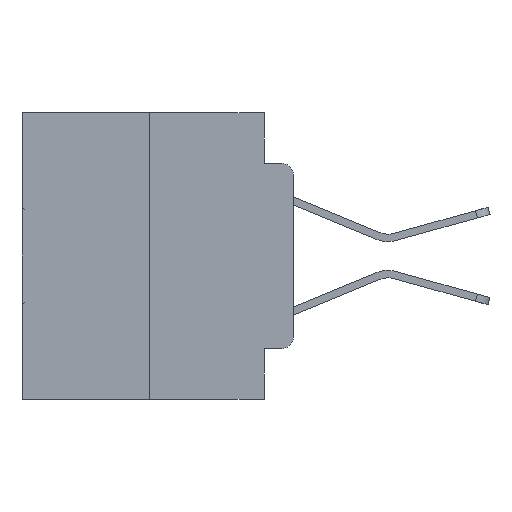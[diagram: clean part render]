
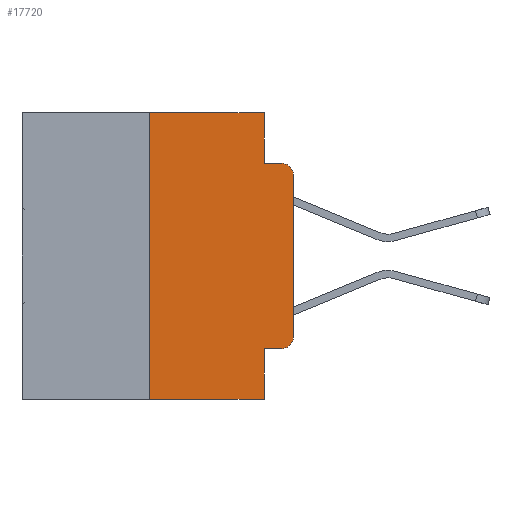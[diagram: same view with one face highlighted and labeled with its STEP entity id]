
A CAD part, left-side view. The second image highlights one B-rep face of the part: STEP entity #17720.
In plain terms, the highlighted planar face has unit normal (-1, 0, 0).
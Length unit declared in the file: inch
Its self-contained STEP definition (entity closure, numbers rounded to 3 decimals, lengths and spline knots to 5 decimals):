
#179 = EDGE_CURVE ( 'NONE', #6998, #27669, #27585, .T. ) ;
#765 = CARTESIAN_POINT ( 'NONE',  ( 0., 0.473, 0. ) ) ;
#1278 = DIRECTION ( 'NONE',  ( 0., -1., 0. ) ) ;
#1785 = CARTESIAN_POINT ( 'NONE',  ( 0., 0.051, -0.0885 ) ) ;
#2516 = VECTOR ( 'NONE', #15667, 39.37008 ) ;
#3267 = DIRECTION ( 'NONE',  ( 1., 0., 0. ) ) ;
#3466 = CARTESIAN_POINT ( 'NONE',  ( 0., 0.051, 0. ) ) ;
#3593 = FACE_OUTER_BOUND ( 'NONE', #20076, .T. ) ;
#4179 = CARTESIAN_POINT ( 'NONE',  ( 0., 0.051, 0. ) ) ;
#4192 = CARTESIAN_POINT ( 'NONE',  ( 0., 0.02, -0.0885 ) ) ;
#4273 = CARTESIAN_POINT ( 'NONE',  ( 0., 0.051, -0.4115 ) ) ;
#4845 = VERTEX_POINT ( 'NONE', #1785 ) ;
#4847 = VECTOR ( 'NONE', #18479, 39.37008 ) ;
#4852 = VERTEX_POINT ( 'NONE', #4273 ) ;
#5198 = ORIENTED_EDGE ( 'NONE', *, *, #9910, .T. ) ;
#5583 = VERTEX_POINT ( 'NONE', #18699 ) ;
#5789 = DIRECTION ( 'NONE',  ( -1., 0., 0. ) ) ;
#6091 = VERTEX_POINT ( 'NONE', #9246 ) ;
#6861 = VERTEX_POINT ( 'NONE', #4192 ) ;
#6998 = VERTEX_POINT ( 'NONE', #18765 ) ;
#7074 = VECTOR ( 'NONE', #29025, 39.37008 ) ;
#7220 = VERTEX_POINT ( 'NONE', #7951 ) ;
#7822 = ORIENTED_EDGE ( 'NONE', *, *, #179, .F. ) ;
#7951 = CARTESIAN_POINT ( 'NONE',  ( 0., 0., -0.3915 ) ) ;
#8272 = LINE ( 'NONE', #4179, #13891 ) ;
#8754 = LINE ( 'NONE', #10656, #20482 ) ;
#9017 = DIRECTION ( 'NONE',  ( 0., 0., -1. ) ) ;
#9246 = CARTESIAN_POINT ( 'NONE',  ( 0., 0., -0.1085 ) ) ;
#9327 = ORIENTED_EDGE ( 'NONE', *, *, #19332, .F. ) ;
#9339 = AXIS2_PLACEMENT_3D ( 'NONE', #765, #3267, #19824 ) ;
#9910 = EDGE_CURVE ( 'NONE', #12800, #7220, #11887, .T. ) ;
#10075 = ORIENTED_EDGE ( 'NONE', *, *, #17796, .F. ) ;
#10470 = VERTEX_POINT ( 'NONE', #27005 ) ;
#10656 = CARTESIAN_POINT ( 'NONE',  ( 0., 0.25, 0. ) ) ;
#11222 = AXIS2_PLACEMENT_3D ( 'NONE', #11922, #28230, #14347 ) ;
#11785 = VECTOR ( 'NONE', #22159, 39.37008 ) ;
#11887 = CIRCLE ( 'NONE', #29180, 0.02 ) ;
#11922 = CARTESIAN_POINT ( 'NONE',  ( 0., 0.02, -0.1085 ) ) ;
#12688 = ORIENTED_EDGE ( 'NONE', *, *, #22464, .F. ) ;
#12800 = VERTEX_POINT ( 'NONE', #26592 ) ;
#13409 = LINE ( 'NONE', #17479, #7074 ) ;
#13891 = VECTOR ( 'NONE', #9017, 39.37008 ) ;
#14347 = DIRECTION ( 'NONE',  ( 0., 0., -1. ) ) ;
#14672 = CARTESIAN_POINT ( 'NONE',  ( 0., 0.473, 0. ) ) ;
#15193 = PLANE ( 'NONE',  #9339 ) ;
#15667 = DIRECTION ( 'NONE',  ( 0., -1., 0. ) ) ;
#15673 = CARTESIAN_POINT ( 'NONE',  ( 0., 0.473, -0.5 ) ) ;
#16267 = EDGE_CURVE ( 'NONE', #4852, #12800, #17466, .T. ) ;
#17466 = LINE ( 'NONE', #30008, #4847 ) ;
#17479 = CARTESIAN_POINT ( 'NONE',  ( 0., 0.051, -0.0885 ) ) ;
#17720 = ADVANCED_FACE ( 'NONE', ( #3593 ), #15193, .F. ) ;
#17796 = EDGE_CURVE ( 'NONE', #4852, #10470, #27877, .T. ) ;
#17934 = VECTOR ( 'NONE', #1278, 39.37008 ) ;
#18011 = LINE ( 'NONE', #19822, #11785 ) ;
#18479 = DIRECTION ( 'NONE',  ( 0., -1., 0. ) ) ;
#18699 = CARTESIAN_POINT ( 'NONE',  ( 0., 0.25, -0.5 ) ) ;
#18765 = CARTESIAN_POINT ( 'NONE',  ( 0., 0.25, 0. ) ) ;
#19332 = EDGE_CURVE ( 'NONE', #5583, #6998, #8754, .T. ) ;
#19822 = CARTESIAN_POINT ( 'NONE',  ( 0., 0., 0. ) ) ;
#19824 = DIRECTION ( 'NONE',  ( 0., 0., -1. ) ) ;
#19922 = CARTESIAN_POINT ( 'NONE',  ( 0., 0.02, -0.3915 ) ) ;
#20076 = EDGE_LOOP ( 'NONE', ( #22857, #29729, #12688, #25051, #7822, #9327, #27960, #10075, #23261, #5198 ) ) ;
#20230 = VECTOR ( 'NONE', #26942, 39.37008 ) ;
#20482 = VECTOR ( 'NONE', #29296, 39.37008 ) ;
#20868 = EDGE_CURVE ( 'NONE', #27669, #4845, #8272, .T. ) ;
#22159 = DIRECTION ( 'NONE',  ( 0., 0., 1. ) ) ;
#22258 = DIRECTION ( 'NONE',  ( 0., 0., -1. ) ) ;
#22464 = EDGE_CURVE ( 'NONE', #4845, #6861, #13409, .T. ) ;
#22857 = ORIENTED_EDGE ( 'NONE', *, *, #25583, .T. ) ;
#23167 = CARTESIAN_POINT ( 'NONE',  ( 0., 0.051, 0. ) ) ;
#23261 = ORIENTED_EDGE ( 'NONE', *, *, #16267, .T. ) ;
#24032 = EDGE_CURVE ( 'NONE', #6091, #6861, #30062, .T. ) ;
#24852 = LINE ( 'NONE', #15673, #17934 ) ;
#25051 = ORIENTED_EDGE ( 'NONE', *, *, #20868, .F. ) ;
#25583 = EDGE_CURVE ( 'NONE', #7220, #6091, #18011, .T. ) ;
#26592 = CARTESIAN_POINT ( 'NONE',  ( 0., 0.02, -0.4115 ) ) ;
#26942 = DIRECTION ( 'NONE',  ( 0., 0., -1. ) ) ;
#27005 = CARTESIAN_POINT ( 'NONE',  ( 0., 0.051, -0.5 ) ) ;
#27526 = EDGE_CURVE ( 'NONE', #5583, #10470, #24852, .T. ) ;
#27585 = LINE ( 'NONE', #14672, #2516 ) ;
#27669 = VERTEX_POINT ( 'NONE', #23167 ) ;
#27877 = LINE ( 'NONE', #3466, #20230 ) ;
#27960 = ORIENTED_EDGE ( 'NONE', *, *, #27526, .T. ) ;
#28230 = DIRECTION ( 'NONE',  ( -1., 0., 0. ) ) ;
#29025 = DIRECTION ( 'NONE',  ( 0., -1., 0. ) ) ;
#29180 = AXIS2_PLACEMENT_3D ( 'NONE', #19922, #5789, #22258 ) ;
#29296 = DIRECTION ( 'NONE',  ( 0., 0., 1. ) ) ;
#29729 = ORIENTED_EDGE ( 'NONE', *, *, #24032, .T. ) ;
#30008 = CARTESIAN_POINT ( 'NONE',  ( 0., 0.051, -0.4115 ) ) ;
#30062 = CIRCLE ( 'NONE', #11222, 0.02 ) ;
